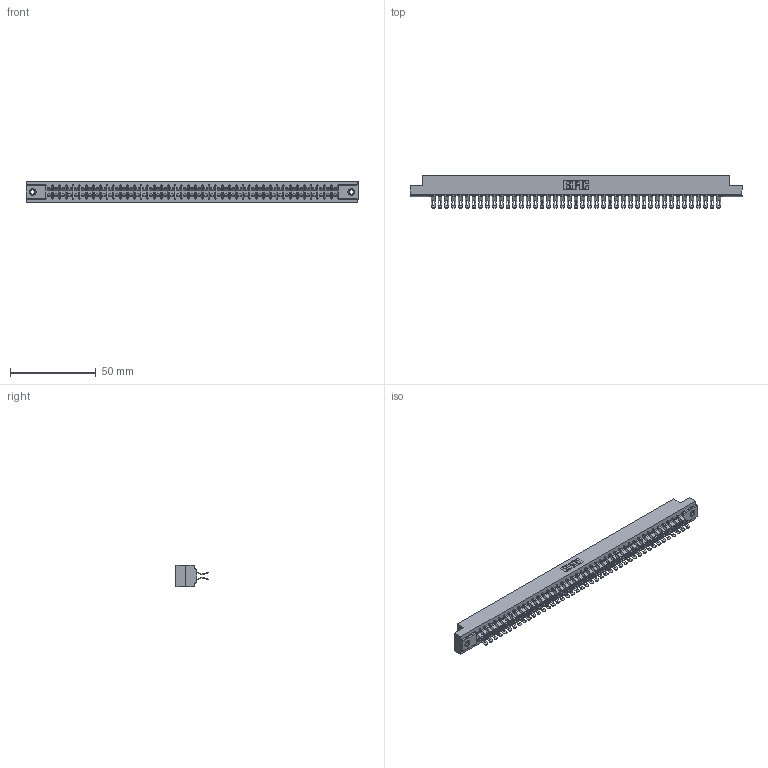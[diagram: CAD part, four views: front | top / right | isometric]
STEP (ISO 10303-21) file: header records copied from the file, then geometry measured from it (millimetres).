
FILE_DESCRIPTION (( 'STEP AP203' ), '1' );
FILE_NAME ('357-086-455-207.STEP', '2020-10-04T06:08:27', ( '' ), ( '' ), 'SwSTEP 2.0', 'SolidWorks 2020', '' );
FILE_SCHEMA (( 'CONFIG_CONTROL_DESIGN' ));
Length unit declared in the file: inch
Products named in the file (4): 345-250-001_345-250-005-103; 357-086-455-207; 307 Part_.156 Dia Mounting Holes; 307-290-001_555
Assembly tree (89 placements, depth 2):
  357-086-455-207
    307 Part_.156 Dia Mounting Holes
    307-290-001_555  x86
    345-250-001_345-250-005-103  x2
Bounding box: 193.4 x 18.75 x 12.7 mm (x, y, z)
Volume: 20815.2 mm3; surface area: 26944.1 mm2
Topology: 89 solids, 89 shells, 5468 faces, 16025 edges, 10442 vertices
Faces by surface type: plane 3026, cylinder 2338, sphere 88, cone 12, torus 4
Entity records: 39838 total; most frequent: CARTESIAN_POINT 6506, ORIENTED_EDGE 6444, DIRECTION 6388, EDGE_CURVE 3222, LINE 2460, VECTOR 2460, VERTEX_POINT 2082, AXIS2_PLACEMENT_3D 1964
